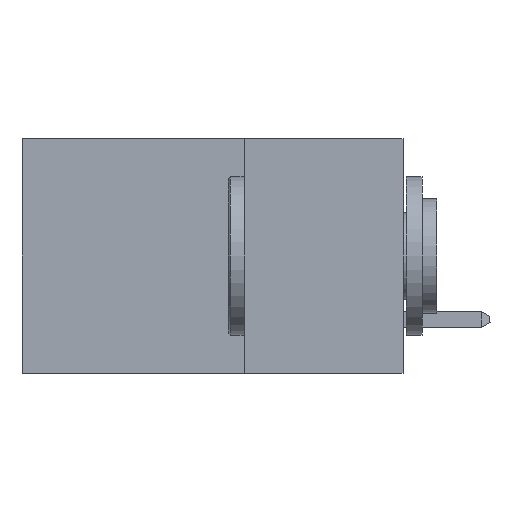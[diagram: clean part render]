
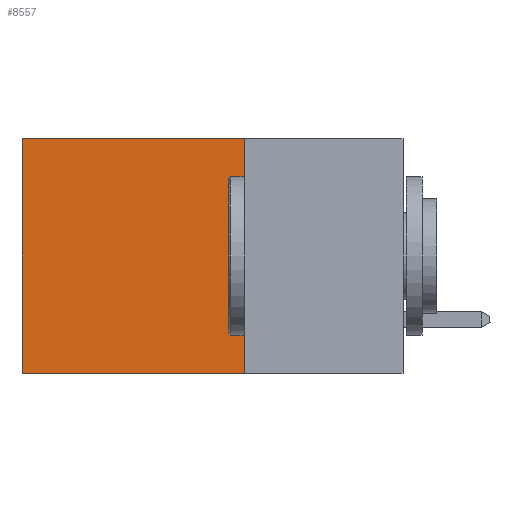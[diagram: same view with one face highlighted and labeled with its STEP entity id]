
A CAD part, left-side view. The second image highlights one B-rep face of the part: STEP entity #8557.
In plain terms, the highlighted planar face has unit normal (-1, 0, 0).
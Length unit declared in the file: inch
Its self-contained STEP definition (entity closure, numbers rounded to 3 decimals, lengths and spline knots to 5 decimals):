
#163 = CARTESIAN_POINT ( 'NONE',  ( 0.2875, 0.25, -0.37 ) ) ;
#640 = LINE ( 'NONE', #3941, #6368 ) ;
#1262 = VECTOR ( 'NONE', #9023, 39.37008 ) ;
#2526 = DIRECTION ( 'NONE',  ( 1., 0., 0. ) ) ;
#2695 = EDGE_CURVE ( 'NONE', #4136, #7002, #4141, .T. ) ;
#3171 = EDGE_CURVE ( 'NONE', #9560, #4136, #3392, .T. ) ;
#3310 = CARTESIAN_POINT ( 'NONE',  ( 0.2875, 0.6, 0. ) ) ;
#3332 = ORIENTED_EDGE ( 'NONE', *, *, #3171, .T. ) ;
#3392 = LINE ( 'NONE', #11481, #4852 ) ;
#3545 = DIRECTION ( 'NONE',  ( 0., 0., -1. ) ) ;
#3941 = CARTESIAN_POINT ( 'NONE',  ( 0.2875, 0.25, -0.37 ) ) ;
#4136 = VERTEX_POINT ( 'NONE', #7286 ) ;
#4141 = LINE ( 'NONE', #3310, #8776 ) ;
#4343 = EDGE_LOOP ( 'NONE', ( #11550, #9412, #9117, #3332 ) ) ;
#4852 = VECTOR ( 'NONE', #7765, 39.37008 ) ;
#5124 = FACE_OUTER_BOUND ( 'NONE', #4343, .T. ) ;
#5604 = EDGE_CURVE ( 'NONE', #10050, #7002, #640, .T. ) ;
#5745 = CARTESIAN_POINT ( 'NONE',  ( 0.2875, 0.25, 0. ) ) ;
#6163 = CARTESIAN_POINT ( 'NONE',  ( 0.2875, 0.6, -0.37 ) ) ;
#6235 = CARTESIAN_POINT ( 'NONE',  ( 0.2875, 0.25, 0. ) ) ;
#6368 = VECTOR ( 'NONE', #7559, 39.37008 ) ;
#6488 = AXIS2_PLACEMENT_3D ( 'NONE', #6235, #2526, #3545 ) ;
#7002 = VERTEX_POINT ( 'NONE', #6163 ) ;
#7286 = CARTESIAN_POINT ( 'NONE',  ( 0.2875, 0.6, 0. ) ) ;
#7559 = DIRECTION ( 'NONE',  ( 0., 1., 0. ) ) ;
#7765 = DIRECTION ( 'NONE',  ( 0., 1., 0. ) ) ;
#7967 = DIRECTION ( 'NONE',  ( 0., 0., -1. ) ) ;
#8066 = EDGE_CURVE ( 'NONE', #9560, #10050, #8754, .T. ) ;
#8557 = ADVANCED_FACE ( 'NONE', ( #5124 ), #8930, .F. ) ;
#8754 = LINE ( 'NONE', #8840, #1262 ) ;
#8776 = VECTOR ( 'NONE', #7967, 39.37008 ) ;
#8840 = CARTESIAN_POINT ( 'NONE',  ( 0.2875, 0.25, 0. ) ) ;
#8930 = PLANE ( 'NONE',  #6488 ) ;
#9023 = DIRECTION ( 'NONE',  ( 0., 0., -1. ) ) ;
#9117 = ORIENTED_EDGE ( 'NONE', *, *, #8066, .F. ) ;
#9412 = ORIENTED_EDGE ( 'NONE', *, *, #5604, .F. ) ;
#9560 = VERTEX_POINT ( 'NONE', #5745 ) ;
#10050 = VERTEX_POINT ( 'NONE', #163 ) ;
#11481 = CARTESIAN_POINT ( 'NONE',  ( 0.2875, 0.25, 0. ) ) ;
#11550 = ORIENTED_EDGE ( 'NONE', *, *, #2695, .T. ) ;
